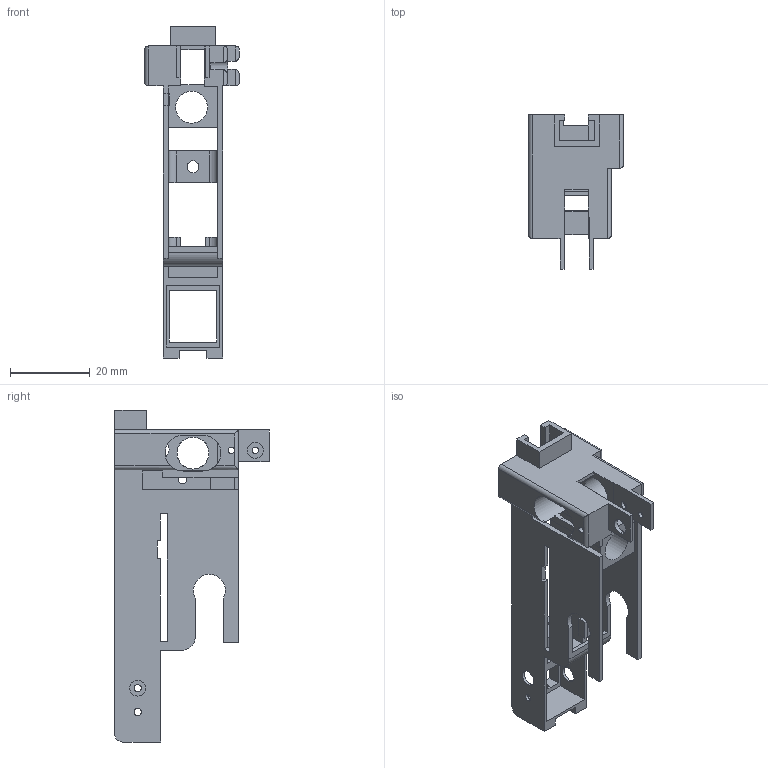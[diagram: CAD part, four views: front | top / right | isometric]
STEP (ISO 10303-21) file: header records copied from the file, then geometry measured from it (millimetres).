
FILE_DESCRIPTION (( 'STEP AP203' ), '1' );
FILE_NAME ('trigger_box.STEP', '2021-12-29T04:21:03', ( '' ), ( '' ), 'SwSTEP 2.0', 'SolidWorks 2015', '' );
FILE_SCHEMA (( 'CONFIG_CONTROL_DESIGN' ));
Length unit declared in the file: millimetre
Products named in the file (1): trigger_box
Bounding box: 23.8 x 38.7 x 83.2 mm (x, y, z)
Volume: 8280.2 mm3; surface area: 11233.3 mm2
Topology: 1 solids, 1 shells, 196 faces, 601 edges, 396 vertices
Faces by surface type: plane 136, cylinder 60
Entity records: 6898 total; most frequent: CARTESIAN_POINT 1296, ORIENTED_EDGE 1202, DIRECTION 1093, EDGE_CURVE 601, LINE 475, VECTOR 475, VERTEX_POINT 396, AXIS2_PLACEMENT_3D 309
